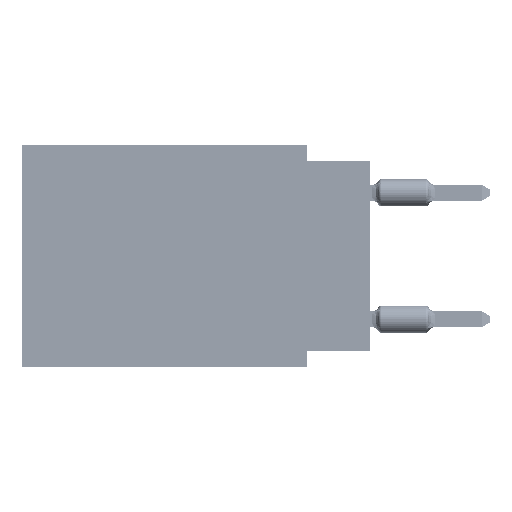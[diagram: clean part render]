
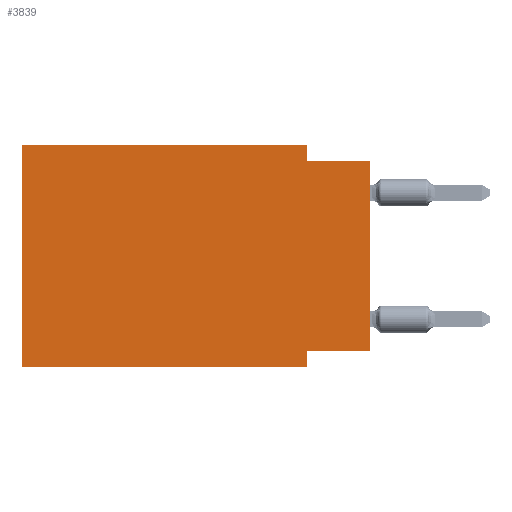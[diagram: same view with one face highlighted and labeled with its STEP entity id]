
A CAD part, left-side view. The second image highlights one B-rep face of the part: STEP entity #3839.
In plain terms, the highlighted planar face has unit normal (-1, 0, 0).
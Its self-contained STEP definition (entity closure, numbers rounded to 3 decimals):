
#1857 = ORIENTED_EDGE ( 'NONE', *, *, #33165, .F. ) ;
#3839 = ADVANCED_FACE ( 'NONE', ( #52970 ), #76097, .F. ) ;
#3960 = DIRECTION ( 'NONE',  ( 0., 0., -1. ) ) ;
#4091 = ORIENTED_EDGE ( 'NONE', *, *, #61971, .F. ) ;
#7308 = VERTEX_POINT ( 'NONE', #23873 ) ;
#9944 = CARTESIAN_POINT ( 'NONE',  ( 0., 13.97, 0. ) ) ;
#10544 = VECTOR ( 'NONE', #3960, 1000. ) ;
#10965 = ORIENTED_EDGE ( 'NONE', *, *, #16056, .F. ) ;
#11355 = ORIENTED_EDGE ( 'NONE', *, *, #23128, .F. ) ;
#12111 = EDGE_CURVE ( 'NONE', #76104, #67491, #47114, .T. ) ;
#12203 = DIRECTION ( 'NONE',  ( 0., 0., 1. ) ) ;
#13356 = ORIENTED_EDGE ( 'NONE', *, *, #73405, .T. ) ;
#16034 = ORIENTED_EDGE ( 'NONE', *, *, #42661, .F. ) ;
#16056 = EDGE_CURVE ( 'NONE', #25210, #20376, #63468, .T. ) ;
#16718 = VECTOR ( 'NONE', #23082, 1000. ) ;
#16936 = DIRECTION ( 'NONE',  ( 0., -1., 0. ) ) ;
#17034 = CARTESIAN_POINT ( 'NONE',  ( 0., 0., -8.255 ) ) ;
#19446 = AXIS2_PLACEMENT_3D ( 'NONE', #9944, #51814, #77246 ) ;
#20376 = VERTEX_POINT ( 'NONE', #26523 ) ;
#21729 = ORIENTED_EDGE ( 'NONE', *, *, #12111, .T. ) ;
#22214 = DIRECTION ( 'NONE',  ( 0., 1., 0. ) ) ;
#22353 = VECTOR ( 'NONE', #38436, 1000. ) ;
#23082 = DIRECTION ( 'NONE',  ( 0., 0., 1. ) ) ;
#23105 = VERTEX_POINT ( 'NONE', #78016 ) ;
#23128 = EDGE_CURVE ( 'NONE', #76104, #68078, #41005, .T. ) ;
#23873 = CARTESIAN_POINT ( 'NONE',  ( 0., 2.54, 0. ) ) ;
#24224 = CARTESIAN_POINT ( 'NONE',  ( 0., 2.54, -8.89 ) ) ;
#25210 = VERTEX_POINT ( 'NONE', #59555 ) ;
#26471 = LINE ( 'NONE', #24224, #22353 ) ;
#26523 = CARTESIAN_POINT ( 'NONE',  ( 0., 0., -0.635 ) ) ;
#30936 = CARTESIAN_POINT ( 'NONE',  ( 0., 2.54, 0. ) ) ;
#33165 = EDGE_CURVE ( 'NONE', #23105, #69423, #52891, .T. ) ;
#36785 = CARTESIAN_POINT ( 'NONE',  ( 0., 13.97, -8.89 ) ) ;
#38198 = ORIENTED_EDGE ( 'NONE', *, *, #40994, .F. ) ;
#38436 = DIRECTION ( 'NONE',  ( 0., 0., -1. ) ) ;
#39166 = CARTESIAN_POINT ( 'NONE',  ( 0., 0., -0.635 ) ) ;
#40994 = EDGE_CURVE ( 'NONE', #7308, #25210, #71951, .T. ) ;
#41005 = LINE ( 'NONE', #65302, #16718 ) ;
#42661 = EDGE_CURVE ( 'NONE', #69423, #67491, #26471, .T. ) ;
#46884 = VECTOR ( 'NONE', #70598, 1000. ) ;
#47114 = LINE ( 'NONE', #52317, #46884 ) ;
#51814 = DIRECTION ( 'NONE',  ( 1., 0., 0. ) ) ;
#52317 = CARTESIAN_POINT ( 'NONE',  ( 0., 13.97, -8.89 ) ) ;
#52891 = LINE ( 'NONE', #17034, #71813 ) ;
#52970 = FACE_OUTER_BOUND ( 'NONE', #78625, .T. ) ;
#57502 = DIRECTION ( 'NONE',  ( 0., -1., 0. ) ) ;
#58139 = VECTOR ( 'NONE', #57502, 1000. ) ;
#59182 = CARTESIAN_POINT ( 'NONE',  ( 0., 2.54, -8.89 ) ) ;
#59555 = CARTESIAN_POINT ( 'NONE',  ( 0., 2.54, -0.635 ) ) ;
#61971 = EDGE_CURVE ( 'NONE', #68078, #7308, #65515, .T. ) ;
#63216 = VECTOR ( 'NONE', #12203, 1000. ) ;
#63468 = LINE ( 'NONE', #39166, #58139 ) ;
#65133 = CARTESIAN_POINT ( 'NONE',  ( 0., 13.97, 0. ) ) ;
#65302 = CARTESIAN_POINT ( 'NONE',  ( 0., 13.97, 0. ) ) ;
#65515 = LINE ( 'NONE', #65133, #68553 ) ;
#66021 = CARTESIAN_POINT ( 'NONE',  ( 0., 0., 0. ) ) ;
#66642 = CARTESIAN_POINT ( 'NONE',  ( 0., 13.97, 0. ) ) ;
#67491 = VERTEX_POINT ( 'NONE', #59182 ) ;
#68078 = VERTEX_POINT ( 'NONE', #66642 ) ;
#68553 = VECTOR ( 'NONE', #16936, 1000. ) ;
#69423 = VERTEX_POINT ( 'NONE', #78376 ) ;
#70598 = DIRECTION ( 'NONE',  ( 0., -1., 0. ) ) ;
#71813 = VECTOR ( 'NONE', #22214, 1000. ) ;
#71951 = LINE ( 'NONE', #30936, #10544 ) ;
#73405 = EDGE_CURVE ( 'NONE', #23105, #20376, #78337, .T. ) ;
#76097 = PLANE ( 'NONE',  #19446 ) ;
#76104 = VERTEX_POINT ( 'NONE', #36785 ) ;
#77246 = DIRECTION ( 'NONE',  ( 0., 0., -1. ) ) ;
#78016 = CARTESIAN_POINT ( 'NONE',  ( 0., 0., -8.255 ) ) ;
#78337 = LINE ( 'NONE', #66021, #63216 ) ;
#78376 = CARTESIAN_POINT ( 'NONE',  ( 0., 2.54, -8.255 ) ) ;
#78625 = EDGE_LOOP ( 'NONE', ( #13356, #10965, #38198, #4091, #11355, #21729, #16034, #1857 ) ) ;
